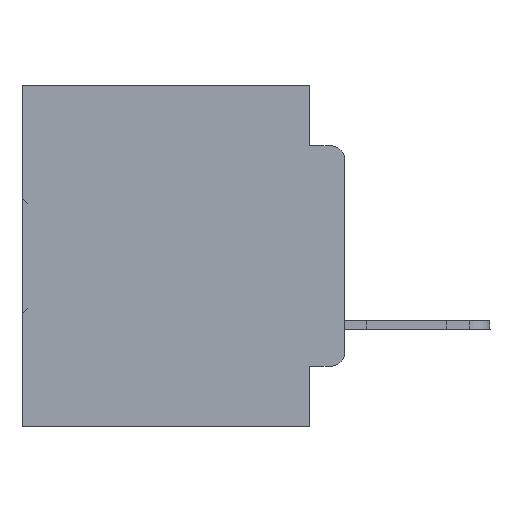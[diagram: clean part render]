
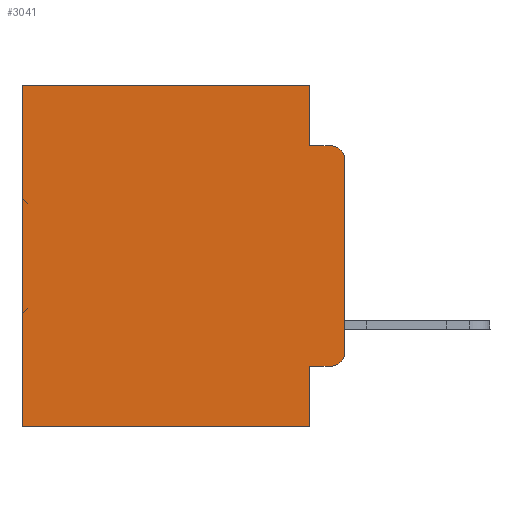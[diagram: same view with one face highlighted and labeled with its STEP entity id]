
A CAD part, left-side view. The second image highlights one B-rep face of the part: STEP entity #3041.
In plain terms, the highlighted planar face has unit normal (-1, 0, 0).
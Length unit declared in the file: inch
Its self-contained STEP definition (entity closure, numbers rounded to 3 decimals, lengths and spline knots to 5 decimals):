
#109 = LINE ( 'NONE', #3192, #18405 ) ;
#745 = ORIENTED_EDGE ( 'NONE', *, *, #25554, .T. ) ;
#1249 = VECTOR ( 'NONE', #21905, 39.37008 ) ;
#1691 = VERTEX_POINT ( 'NONE', #12427 ) ;
#3041 = ADVANCED_FACE ( 'NONE', ( #36593 ), #10260, .F. ) ;
#3192 = CARTESIAN_POINT ( 'NONE',  ( 0.298, 0.051, 0. ) ) ;
#3216 = ORIENTED_EDGE ( 'NONE', *, *, #13418, .F. ) ;
#3364 = VERTEX_POINT ( 'NONE', #27909 ) ;
#3448 = VERTEX_POINT ( 'NONE', #22321 ) ;
#4185 = DIRECTION ( 'NONE',  ( 0., 0., -1. ) ) ;
#4774 = ORIENTED_EDGE ( 'NONE', *, *, #15144, .F. ) ;
#5036 = LINE ( 'NONE', #22716, #28872 ) ;
#5133 = VERTEX_POINT ( 'NONE', #10553 ) ;
#5499 = CIRCLE ( 'NONE', #37413, 0.02 ) ;
#6108 = DIRECTION ( 'NONE',  ( 0., 0., -1. ) ) ;
#6541 = EDGE_CURVE ( 'NONE', #3448, #10818, #28504, .T. ) ;
#6757 = EDGE_CURVE ( 'NONE', #34404, #30377, #21529, .T. ) ;
#6940 = DIRECTION ( 'NONE',  ( 0., -1., 0. ) ) ;
#7260 = ORIENTED_EDGE ( 'NONE', *, *, #21312, .F. ) ;
#8603 = DIRECTION ( 'NONE',  ( -1., 0., 0. ) ) ;
#8645 = VECTOR ( 'NONE', #6940, 39.37008 ) ;
#10260 = PLANE ( 'NONE',  #17409 ) ;
#10553 = CARTESIAN_POINT ( 'NONE',  ( 0.298, 0.473, 0. ) ) ;
#10758 = LINE ( 'NONE', #19416, #28929 ) ;
#10818 = VERTEX_POINT ( 'NONE', #26859 ) ;
#11414 = DIRECTION ( 'NONE',  ( 0., 0., -1. ) ) ;
#12427 = CARTESIAN_POINT ( 'NONE',  ( 0.298, 0., -0.3915 ) ) ;
#12810 = VECTOR ( 'NONE', #31897, 39.37008 ) ;
#13418 = EDGE_CURVE ( 'NONE', #3364, #18115, #25559, .T. ) ;
#14518 = EDGE_CURVE ( 'NONE', #34404, #3364, #109, .T. ) ;
#14761 = CARTESIAN_POINT ( 'NONE',  ( 0.298, 0.02, -0.1085 ) ) ;
#14811 = CARTESIAN_POINT ( 'NONE',  ( 0.298, 0.02, -0.3915 ) ) ;
#14821 = CARTESIAN_POINT ( 'NONE',  ( 0.298, 0., -0.1085 ) ) ;
#15144 = EDGE_CURVE ( 'NONE', #10818, #17063, #5036, .T. ) ;
#16527 = DIRECTION ( 'NONE',  ( 0., 0., -1. ) ) ;
#16780 = EDGE_CURVE ( 'NONE', #3448, #5133, #24807, .T. ) ;
#17063 = VERTEX_POINT ( 'NONE', #35724 ) ;
#17153 = DIRECTION ( 'NONE',  ( 0., 0., -1. ) ) ;
#17409 = AXIS2_PLACEMENT_3D ( 'NONE', #37915, #23706, #11414 ) ;
#17613 = DIRECTION ( 'NONE',  ( 0., 0., -1. ) ) ;
#17885 = VECTOR ( 'NONE', #17153, 39.37008 ) ;
#18115 = VERTEX_POINT ( 'NONE', #18506 ) ;
#18405 = VECTOR ( 'NONE', #17613, 39.37008 ) ;
#18506 = CARTESIAN_POINT ( 'NONE',  ( 0.298, 0.473, -0.5 ) ) ;
#18979 = AXIS2_PLACEMENT_3D ( 'NONE', #14761, #8603, #6108 ) ;
#19416 = CARTESIAN_POINT ( 'NONE',  ( 0.298, 0., 0. ) ) ;
#19663 = VERTEX_POINT ( 'NONE', #14821 ) ;
#19938 = CARTESIAN_POINT ( 'NONE',  ( 0.298, 0.02, -0.4115 ) ) ;
#21312 = EDGE_CURVE ( 'NONE', #19663, #1691, #10758, .T. ) ;
#21529 = LINE ( 'NONE', #33457, #8645 ) ;
#21905 = DIRECTION ( 'NONE',  ( 0., 1., 0. ) ) ;
#22048 = ORIENTED_EDGE ( 'NONE', *, *, #14518, .F. ) ;
#22095 = CARTESIAN_POINT ( 'NONE',  ( 0.298, 0., 0. ) ) ;
#22321 = CARTESIAN_POINT ( 'NONE',  ( 0.298, 0.051, 0. ) ) ;
#22716 = CARTESIAN_POINT ( 'NONE',  ( 0.298, 0.051, -0.0885 ) ) ;
#23706 = DIRECTION ( 'NONE',  ( 1., 0., 0. ) ) ;
#23783 = ORIENTED_EDGE ( 'NONE', *, *, #31831, .T. ) ;
#24807 = LINE ( 'NONE', #22095, #1249 ) ;
#25088 = ORIENTED_EDGE ( 'NONE', *, *, #16780, .T. ) ;
#25554 = EDGE_CURVE ( 'NONE', #5133, #18115, #27630, .T. ) ;
#25559 = LINE ( 'NONE', #34778, #12810 ) ;
#26859 = CARTESIAN_POINT ( 'NONE',  ( 0.298, 0.051, -0.0885 ) ) ;
#27630 = LINE ( 'NONE', #28004, #34012 ) ;
#27909 = CARTESIAN_POINT ( 'NONE',  ( 0.298, 0.051, -0.5 ) ) ;
#28004 = CARTESIAN_POINT ( 'NONE',  ( 0.298, 0.473, 0. ) ) ;
#28504 = LINE ( 'NONE', #34445, #17885 ) ;
#28872 = VECTOR ( 'NONE', #37110, 39.37008 ) ;
#28929 = VECTOR ( 'NONE', #16527, 39.37008 ) ;
#30002 = DIRECTION ( 'NONE',  ( 0., 0., -1. ) ) ;
#30060 = CARTESIAN_POINT ( 'NONE',  ( 0.298, 0.051, -0.4115 ) ) ;
#30377 = VERTEX_POINT ( 'NONE', #19938 ) ;
#30914 = ORIENTED_EDGE ( 'NONE', *, *, #6757, .T. ) ;
#31156 = EDGE_LOOP ( 'NONE', ( #7260, #23783, #4774, #33254, #25088, #745, #3216, #22048, #30914, #32564 ) ) ;
#31831 = EDGE_CURVE ( 'NONE', #19663, #17063, #33701, .T. ) ;
#31897 = DIRECTION ( 'NONE',  ( 0., 1., 0. ) ) ;
#32564 = ORIENTED_EDGE ( 'NONE', *, *, #33271, .T. ) ;
#33049 = DIRECTION ( 'NONE',  ( -1., 0., 0. ) ) ;
#33254 = ORIENTED_EDGE ( 'NONE', *, *, #6541, .F. ) ;
#33271 = EDGE_CURVE ( 'NONE', #30377, #1691, #5499, .T. ) ;
#33457 = CARTESIAN_POINT ( 'NONE',  ( 0.298, 0.051, -0.4115 ) ) ;
#33701 = CIRCLE ( 'NONE', #18979, 0.02 ) ;
#34012 = VECTOR ( 'NONE', #4185, 39.37008 ) ;
#34404 = VERTEX_POINT ( 'NONE', #30060 ) ;
#34445 = CARTESIAN_POINT ( 'NONE',  ( 0.298, 0.051, 0. ) ) ;
#34778 = CARTESIAN_POINT ( 'NONE',  ( 0.298, 0., -0.5 ) ) ;
#35724 = CARTESIAN_POINT ( 'NONE',  ( 0.298, 0.02, -0.0885 ) ) ;
#36593 = FACE_OUTER_BOUND ( 'NONE', #31156, .T. ) ;
#37110 = DIRECTION ( 'NONE',  ( 0., -1., 0. ) ) ;
#37413 = AXIS2_PLACEMENT_3D ( 'NONE', #14811, #33049, #30002 ) ;
#37915 = CARTESIAN_POINT ( 'NONE',  ( 0.298, 0., 0. ) ) ;
